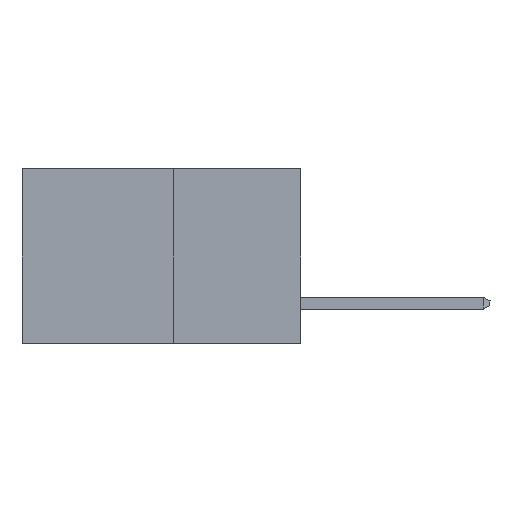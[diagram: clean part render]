
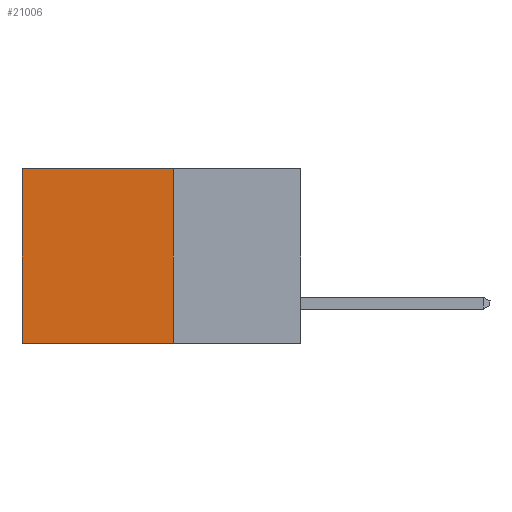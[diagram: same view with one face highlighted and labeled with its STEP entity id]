
A CAD part, left-side view. The second image highlights one B-rep face of the part: STEP entity #21006.
In plain terms, the highlighted planar face has unit normal (-1, 0, 0).
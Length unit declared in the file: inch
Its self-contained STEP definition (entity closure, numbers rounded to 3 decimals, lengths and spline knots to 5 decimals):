
#122 = VERTEX_POINT ( 'NONE', #7359 ) ;
#488 = LINE ( 'NONE', #17089, #19280 ) ;
#1107 = EDGE_CURVE ( 'NONE', #4600, #16778, #10029, .T. ) ;
#2261 = EDGE_CURVE ( 'NONE', #3204, #16778, #488, .T. ) ;
#2813 = EDGE_CURVE ( 'NONE', #122, #4600, #21130, .T. ) ;
#3204 = VERTEX_POINT ( 'NONE', #21110 ) ;
#3475 = CARTESIAN_POINT ( 'NONE',  ( 0.277, 0.27, -0.37 ) ) ;
#3955 = DIRECTION ( 'NONE',  ( 1., 0., 0. ) ) ;
#4283 = ORIENTED_EDGE ( 'NONE', *, *, #13296, .T. ) ;
#4600 = VERTEX_POINT ( 'NONE', #3475 ) ;
#5078 = LINE ( 'NONE', #11464, #18094 ) ;
#5223 = AXIS2_PLACEMENT_3D ( 'NONE', #14532, #3955, #16367 ) ;
#5644 = ORIENTED_EDGE ( 'NONE', *, *, #2261, .T. ) ;
#6285 = CARTESIAN_POINT ( 'NONE',  ( 0.277, 0.27, -0.37 ) ) ;
#7359 = CARTESIAN_POINT ( 'NONE',  ( 0.277, 0.27, 0. ) ) ;
#8846 = VECTOR ( 'NONE', #12049, 39.37008 ) ;
#9628 = FACE_OUTER_BOUND ( 'NONE', #13109, .T. ) ;
#10029 = LINE ( 'NONE', #6285, #14719 ) ;
#11464 = CARTESIAN_POINT ( 'NONE',  ( 0.277, 0.27, 0. ) ) ;
#12049 = DIRECTION ( 'NONE',  ( 0., 0., -1. ) ) ;
#12095 = ORIENTED_EDGE ( 'NONE', *, *, #1107, .F. ) ;
#12512 = DIRECTION ( 'NONE',  ( 0., 1., 0. ) ) ;
#13109 = EDGE_LOOP ( 'NONE', ( #5644, #12095, #20021, #4283 ) ) ;
#13296 = EDGE_CURVE ( 'NONE', #122, #3204, #5078, .T. ) ;
#14532 = CARTESIAN_POINT ( 'NONE',  ( 0.277, 0.27, -0.37 ) ) ;
#14719 = VECTOR ( 'NONE', #12512, 39.37008 ) ;
#16367 = DIRECTION ( 'NONE',  ( 0., 0., -1. ) ) ;
#16778 = VERTEX_POINT ( 'NONE', #18082 ) ;
#17089 = CARTESIAN_POINT ( 'NONE',  ( 0.277, 0.59, -0.37 ) ) ;
#17305 = CARTESIAN_POINT ( 'NONE',  ( 0.277, 0.27, -0.37 ) ) ;
#18082 = CARTESIAN_POINT ( 'NONE',  ( 0.277, 0.59, -0.37 ) ) ;
#18094 = VECTOR ( 'NONE', #21875, 39.37008 ) ;
#19280 = VECTOR ( 'NONE', #21015, 39.37008 ) ;
#20021 = ORIENTED_EDGE ( 'NONE', *, *, #2813, .F. ) ;
#21006 = ADVANCED_FACE ( 'NONE', ( #9628 ), #21516, .F. ) ;
#21015 = DIRECTION ( 'NONE',  ( 0., 0., -1. ) ) ;
#21110 = CARTESIAN_POINT ( 'NONE',  ( 0.277, 0.59, 0. ) ) ;
#21130 = LINE ( 'NONE', #17305, #8846 ) ;
#21516 = PLANE ( 'NONE',  #5223 ) ;
#21875 = DIRECTION ( 'NONE',  ( 0., 1., 0. ) ) ;
